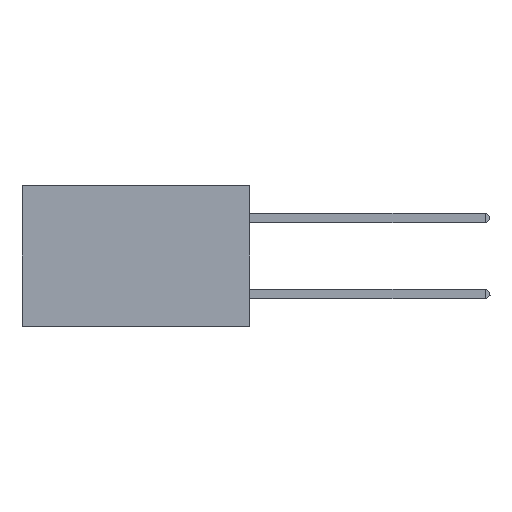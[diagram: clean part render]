
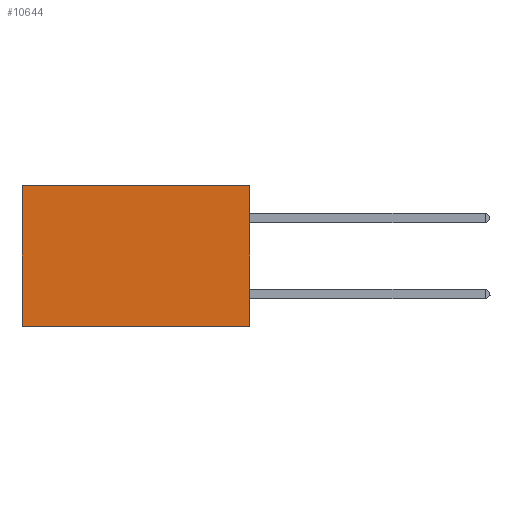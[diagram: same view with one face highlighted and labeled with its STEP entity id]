
A CAD part, left-side view. The second image highlights one B-rep face of the part: STEP entity #10644.
In plain terms, the highlighted planar face has unit normal (-1, 0, 0).
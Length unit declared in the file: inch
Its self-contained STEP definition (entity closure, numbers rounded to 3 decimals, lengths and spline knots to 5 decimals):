
#577 = CARTESIAN_POINT ( 'NONE',  ( 0.2875, 0.6, -0.37 ) ) ;
#677 = DIRECTION ( 'NONE',  ( 1., 0., 0. ) ) ;
#1168 = VERTEX_POINT ( 'NONE', #9532 ) ;
#1234 = EDGE_LOOP ( 'NONE', ( #15799, #18291, #3713, #19432 ) ) ;
#2694 = CARTESIAN_POINT ( 'NONE',  ( 0.2875, 0.6, 0. ) ) ;
#3388 = CARTESIAN_POINT ( 'NONE',  ( 0.2875, 0., -0.37 ) ) ;
#3713 = ORIENTED_EDGE ( 'NONE', *, *, #7248, .F. ) ;
#4375 = DIRECTION ( 'NONE',  ( 0., 0., -1. ) ) ;
#5089 = CARTESIAN_POINT ( 'NONE',  ( 0.2875, 0., 0. ) ) ;
#5971 = VECTOR ( 'NONE', #14477, 39.37008 ) ;
#6879 = VERTEX_POINT ( 'NONE', #577 ) ;
#7248 = EDGE_CURVE ( 'NONE', #1168, #17198, #19685, .T. ) ;
#7589 = EDGE_CURVE ( 'NONE', #13498, #6879, #11053, .T. ) ;
#8413 = PLANE ( 'NONE',  #13227 ) ;
#9034 = DIRECTION ( 'NONE',  ( 0., 0., -1. ) ) ;
#9417 = LINE ( 'NONE', #11434, #5971 ) ;
#9532 = CARTESIAN_POINT ( 'NONE',  ( 0.2875, 0., 0. ) ) ;
#9659 = CARTESIAN_POINT ( 'NONE',  ( 0.2875, 0.6, 0. ) ) ;
#10644 = ADVANCED_FACE ( 'NONE', ( #19595 ), #8413, .F. ) ;
#11053 = LINE ( 'NONE', #2694, #12546 ) ;
#11434 = CARTESIAN_POINT ( 'NONE',  ( 0.2875, 0., 0. ) ) ;
#11643 = DIRECTION ( 'NONE',  ( 0., 0., -1. ) ) ;
#12546 = VECTOR ( 'NONE', #9034, 39.37008 ) ;
#13227 = AXIS2_PLACEMENT_3D ( 'NONE', #5089, #677, #11643 ) ;
#13274 = DIRECTION ( 'NONE',  ( 0., 1., 0. ) ) ;
#13498 = VERTEX_POINT ( 'NONE', #9659 ) ;
#13654 = LINE ( 'NONE', #18301, #20033 ) ;
#13880 = CARTESIAN_POINT ( 'NONE',  ( 0.2875, 0., 0. ) ) ;
#14477 = DIRECTION ( 'NONE',  ( 0., 1., 0. ) ) ;
#15507 = VECTOR ( 'NONE', #4375, 39.37008 ) ;
#15799 = ORIENTED_EDGE ( 'NONE', *, *, #7589, .T. ) ;
#17198 = VERTEX_POINT ( 'NONE', #3388 ) ;
#18291 = ORIENTED_EDGE ( 'NONE', *, *, #18348, .F. ) ;
#18301 = CARTESIAN_POINT ( 'NONE',  ( 0.2875, 0., -0.37 ) ) ;
#18348 = EDGE_CURVE ( 'NONE', #17198, #6879, #13654, .T. ) ;
#18413 = EDGE_CURVE ( 'NONE', #1168, #13498, #9417, .T. ) ;
#19432 = ORIENTED_EDGE ( 'NONE', *, *, #18413, .T. ) ;
#19595 = FACE_OUTER_BOUND ( 'NONE', #1234, .T. ) ;
#19685 = LINE ( 'NONE', #13880, #15507 ) ;
#20033 = VECTOR ( 'NONE', #13274, 39.37008 ) ;
